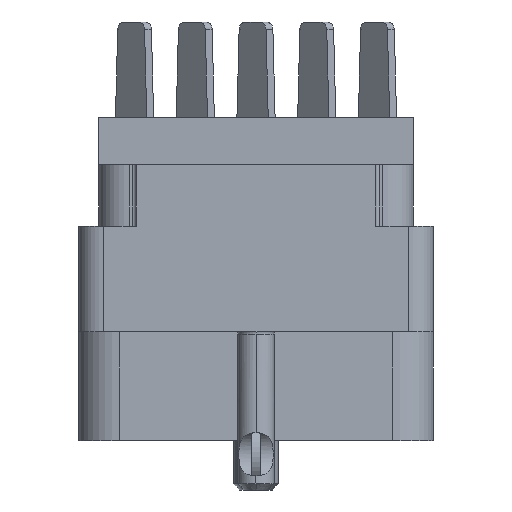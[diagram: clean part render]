
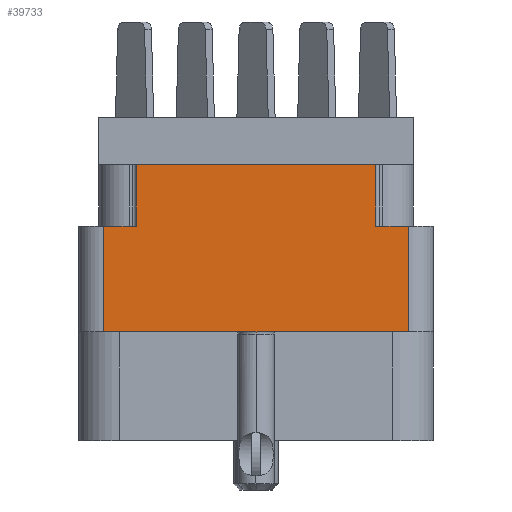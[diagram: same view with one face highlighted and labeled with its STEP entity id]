
A CAD part, left-side view. The second image highlights one B-rep face of the part: STEP entity #39733.
In plain terms, the highlighted planar face has unit normal (-1, 0, 0).
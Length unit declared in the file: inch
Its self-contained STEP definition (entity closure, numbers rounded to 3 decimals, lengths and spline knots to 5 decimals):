
#372 = CARTESIAN_POINT ( 'NONE',  ( -1., 0.438, -0.268 ) ) ;
#1722 = CARTESIAN_POINT ( 'NONE',  ( -1., 0.296, -0.268 ) ) ;
#2879 = VECTOR ( 'NONE', #8807, 39.37008 ) ;
#3140 = EDGE_LOOP ( 'NONE', ( #10673, #36057, #5365, #28648, #31783, #8548, #36298, #12343 ) ) ;
#4811 = CARTESIAN_POINT ( 'NONE',  ( -1., 0.296, -0.268 ) ) ;
#5056 = FACE_OUTER_BOUND ( 'NONE', #3140, .T. ) ;
#5295 = CARTESIAN_POINT ( 'NONE',  ( -1., -0.296, -0.268 ) ) ;
#5365 = ORIENTED_EDGE ( 'NONE', *, *, #9233, .T. ) ;
#6089 = EDGE_CURVE ( 'NONE', #9373, #32513, #43005, .T. ) ;
#6272 = VECTOR ( 'NONE', #31674, 39.37008 ) ;
#6620 = CARTESIAN_POINT ( 'NONE',  ( -1., -0.296, -0.268 ) ) ;
#7812 = AXIS2_PLACEMENT_3D ( 'NONE', #39820, #29183, #22910 ) ;
#8003 = EDGE_CURVE ( 'NONE', #32513, #35450, #45397, .T. ) ;
#8548 = ORIENTED_EDGE ( 'NONE', *, *, #17618, .F. ) ;
#8807 = DIRECTION ( 'NONE',  ( 0., -1., 0. ) ) ;
#9233 = EDGE_CURVE ( 'NONE', #34276, #38967, #33412, .T. ) ;
#9373 = VERTEX_POINT ( 'NONE', #9944 ) ;
#9704 = DIRECTION ( 'NONE',  ( 0., -1., 0. ) ) ;
#9944 = CARTESIAN_POINT ( 'NONE',  ( -1., 0.376, -0.529 ) ) ;
#10673 = ORIENTED_EDGE ( 'NONE', *, *, #6089, .F. ) ;
#11070 = EDGE_CURVE ( 'NONE', #11782, #14922, #23387, .T. ) ;
#11782 = VERTEX_POINT ( 'NONE', #30748 ) ;
#12343 = ORIENTED_EDGE ( 'NONE', *, *, #8003, .F. ) ;
#14922 = VERTEX_POINT ( 'NONE', #30836 ) ;
#17618 = EDGE_CURVE ( 'NONE', #43935, #14922, #44802, .T. ) ;
#18230 = DIRECTION ( 'NONE',  ( 0., 0., 1. ) ) ;
#18950 = DIRECTION ( 'NONE',  ( 0., 0., 1. ) ) ;
#19741 = EDGE_CURVE ( 'NONE', #35450, #43935, #22428, .T. ) ;
#20006 = CARTESIAN_POINT ( 'NONE',  ( -1., -0.376, -0.529 ) ) ;
#21304 = VECTOR ( 'NONE', #23199, 39.37008 ) ;
#21530 = VECTOR ( 'NONE', #45022, 39.37008 ) ;
#22241 = VECTOR ( 'NONE', #44229, 39.37008 ) ;
#22428 = LINE ( 'NONE', #4811, #43960 ) ;
#22910 = DIRECTION ( 'NONE',  ( 0., 0., 1. ) ) ;
#23199 = DIRECTION ( 'NONE',  ( 0., 0., 1. ) ) ;
#23387 = LINE ( 'NONE', #5295, #22241 ) ;
#26464 = LINE ( 'NONE', #40329, #2879 ) ;
#27687 = CARTESIAN_POINT ( 'NONE',  ( -1., 0.438, -0.117 ) ) ;
#28216 = LINE ( 'NONE', #6620, #6272 ) ;
#28648 = ORIENTED_EDGE ( 'NONE', *, *, #33151, .F. ) ;
#29183 = DIRECTION ( 'NONE',  ( -1., 0., 0. ) ) ;
#30748 = CARTESIAN_POINT ( 'NONE',  ( -1., -0.296, -0.268 ) ) ;
#30836 = CARTESIAN_POINT ( 'NONE',  ( -1., -0.296, -0.117 ) ) ;
#31674 = DIRECTION ( 'NONE',  ( 0., -1., 0. ) ) ;
#31783 = ORIENTED_EDGE ( 'NONE', *, *, #11070, .T. ) ;
#32513 = VERTEX_POINT ( 'NONE', #37765 ) ;
#33075 = CARTESIAN_POINT ( 'NONE',  ( -1., 0.376, -0.798 ) ) ;
#33151 = EDGE_CURVE ( 'NONE', #11782, #38967, #28216, .T. ) ;
#33412 = LINE ( 'NONE', #43810, #21304 ) ;
#34276 = VERTEX_POINT ( 'NONE', #20006 ) ;
#35450 = VERTEX_POINT ( 'NONE', #1722 ) ;
#36057 = ORIENTED_EDGE ( 'NONE', *, *, #38032, .T. ) ;
#36298 = ORIENTED_EDGE ( 'NONE', *, *, #19741, .F. ) ;
#37377 = VECTOR ( 'NONE', #9704, 39.37008 ) ;
#37765 = CARTESIAN_POINT ( 'NONE',  ( -1., 0.376, -0.268 ) ) ;
#38032 = EDGE_CURVE ( 'NONE', #9373, #34276, #26464, .T. ) ;
#38967 = VERTEX_POINT ( 'NONE', #44163 ) ;
#39733 = ADVANCED_FACE ( 'NONE', ( #5056 ), #43750, .T. ) ;
#39820 = CARTESIAN_POINT ( 'NONE',  ( -1., -0.376, -0.798 ) ) ;
#40329 = CARTESIAN_POINT ( 'NONE',  ( -1., 0., -0.529 ) ) ;
#40602 = VECTOR ( 'NONE', #18230, 39.37008 ) ;
#43005 = LINE ( 'NONE', #33075, #40602 ) ;
#43750 = PLANE ( 'NONE',  #7812 ) ;
#43810 = CARTESIAN_POINT ( 'NONE',  ( -1., -0.376, -0.798 ) ) ;
#43935 = VERTEX_POINT ( 'NONE', #44806 ) ;
#43960 = VECTOR ( 'NONE', #18950, 39.37008 ) ;
#44163 = CARTESIAN_POINT ( 'NONE',  ( -1., -0.376, -0.268 ) ) ;
#44229 = DIRECTION ( 'NONE',  ( 0., 0., 1. ) ) ;
#44802 = LINE ( 'NONE', #27687, #21530 ) ;
#44806 = CARTESIAN_POINT ( 'NONE',  ( -1., 0.296, -0.117 ) ) ;
#45022 = DIRECTION ( 'NONE',  ( 0., -1., 0. ) ) ;
#45397 = LINE ( 'NONE', #372, #37377 ) ;
